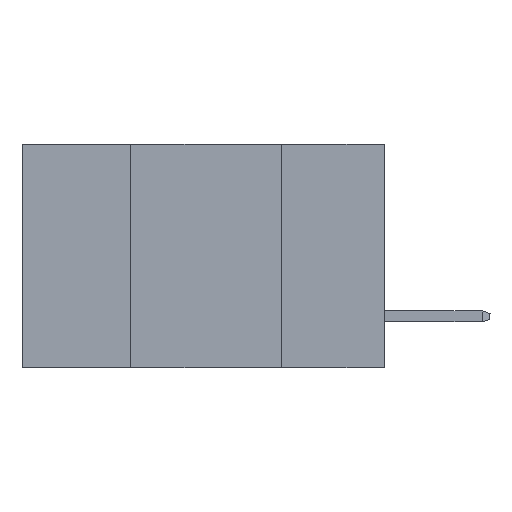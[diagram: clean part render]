
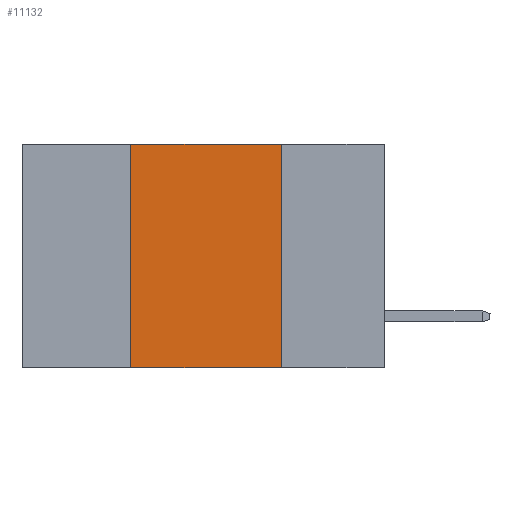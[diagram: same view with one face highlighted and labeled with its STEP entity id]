
A CAD part, left-side view. The second image highlights one B-rep face of the part: STEP entity #11132.
In plain terms, the highlighted planar face has unit normal (-1, 0, 0).
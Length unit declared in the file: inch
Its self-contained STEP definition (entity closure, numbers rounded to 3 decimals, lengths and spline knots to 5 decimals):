
#696 = ORIENTED_EDGE ( 'NONE', *, *, #5725, .T. ) ;
#702 = LINE ( 'NONE', #9497, #801 ) ;
#801 = VECTOR ( 'NONE', #1432, 39.37008 ) ;
#816 = FACE_OUTER_BOUND ( 'NONE', #11164, .T. ) ;
#1291 = VERTEX_POINT ( 'NONE', #5627 ) ;
#1432 = DIRECTION ( 'NONE',  ( 0., 0., -1. ) ) ;
#1727 = CARTESIAN_POINT ( 'NONE',  ( 0., 0.42, -0.37 ) ) ;
#1772 = DIRECTION ( 'NONE',  ( 1., 0., 0. ) ) ;
#2687 = CARTESIAN_POINT ( 'NONE',  ( 0., 0.42, -0.37 ) ) ;
#3426 = VERTEX_POINT ( 'NONE', #2687 ) ;
#3666 = DIRECTION ( 'NONE',  ( 0., 0., -1. ) ) ;
#4157 = VERTEX_POINT ( 'NONE', #7916 ) ;
#4461 = PLANE ( 'NONE',  #8940 ) ;
#5228 = DIRECTION ( 'NONE',  ( 0., -1., 0. ) ) ;
#5326 = ORIENTED_EDGE ( 'NONE', *, *, #9665, .F. ) ;
#5435 = EDGE_CURVE ( 'NONE', #9032, #1291, #7586, .T. ) ;
#5627 = CARTESIAN_POINT ( 'NONE',  ( 0., 0.17, 0. ) ) ;
#5725 = EDGE_CURVE ( 'NONE', #3426, #4157, #7225, .T. ) ;
#6951 = VECTOR ( 'NONE', #5228, 39.37008 ) ;
#7225 = LINE ( 'NONE', #8866, #6951 ) ;
#7586 = LINE ( 'NONE', #9227, #11463 ) ;
#7916 = CARTESIAN_POINT ( 'NONE',  ( 0., 0.17, -0.37 ) ) ;
#7953 = VECTOR ( 'NONE', #8140, 39.37008 ) ;
#7974 = LINE ( 'NONE', #1727, #7953 ) ;
#8140 = DIRECTION ( 'NONE',  ( 0., 0., 1. ) ) ;
#8580 = ORIENTED_EDGE ( 'NONE', *, *, #9302, .F. ) ;
#8866 = CARTESIAN_POINT ( 'NONE',  ( 0., 0.6, -0.37 ) ) ;
#8940 = AXIS2_PLACEMENT_3D ( 'NONE', #9843, #1772, #3666 ) ;
#9032 = VERTEX_POINT ( 'NONE', #11102 ) ;
#9049 = ORIENTED_EDGE ( 'NONE', *, *, #5435, .F. ) ;
#9227 = CARTESIAN_POINT ( 'NONE',  ( 0., 0.6, 0. ) ) ;
#9302 = EDGE_CURVE ( 'NONE', #3426, #9032, #7974, .T. ) ;
#9497 = CARTESIAN_POINT ( 'NONE',  ( 0., 0.17, -0.37 ) ) ;
#9665 = EDGE_CURVE ( 'NONE', #1291, #4157, #702, .T. ) ;
#9843 = CARTESIAN_POINT ( 'NONE',  ( 0., 0.6, 0. ) ) ;
#11102 = CARTESIAN_POINT ( 'NONE',  ( 0., 0.42, 0. ) ) ;
#11132 = ADVANCED_FACE ( 'NONE', ( #816 ), #4461, .F. ) ;
#11159 = DIRECTION ( 'NONE',  ( 0., -1., 0. ) ) ;
#11164 = EDGE_LOOP ( 'NONE', ( #5326, #9049, #8580, #696 ) ) ;
#11463 = VECTOR ( 'NONE', #11159, 39.37008 ) ;
